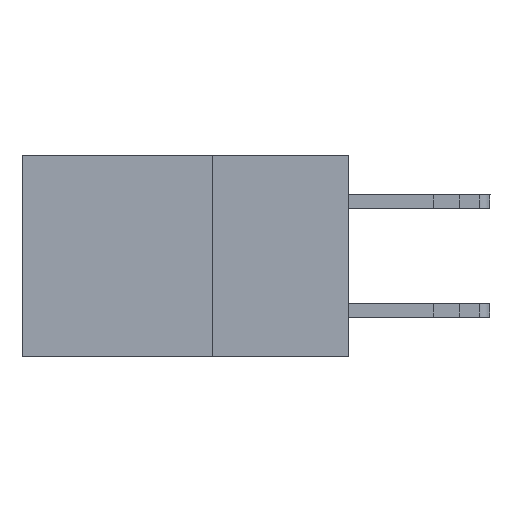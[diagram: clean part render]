
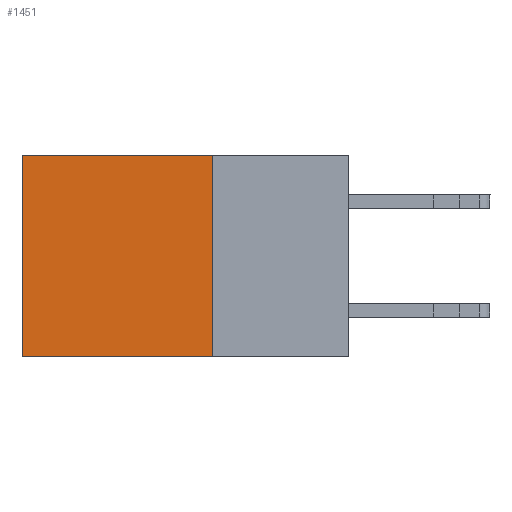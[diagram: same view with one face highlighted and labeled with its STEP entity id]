
A CAD part, left-side view. The second image highlights one B-rep face of the part: STEP entity #1451.
In plain terms, the highlighted planar face has unit normal (-1, 0, 0).
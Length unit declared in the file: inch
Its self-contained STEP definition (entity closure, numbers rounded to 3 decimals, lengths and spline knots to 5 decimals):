
#61 = VERTEX_POINT ( 'NONE', #7611 ) ;
#234 = VECTOR ( 'NONE', #950, 39.37008 ) ;
#636 = EDGE_LOOP ( 'NONE', ( #12539, #14292, #8505, #3517 ) ) ;
#950 = DIRECTION ( 'NONE',  ( 0., 0., -1. ) ) ;
#1048 = VECTOR ( 'NONE', #4160, 39.37008 ) ;
#1451 = ADVANCED_FACE ( 'NONE', ( #7456 ), #11274, .F. ) ;
#1726 = CARTESIAN_POINT ( 'NONE',  ( 0.298, 0.6, -0.37 ) ) ;
#2780 = VERTEX_POINT ( 'NONE', #1726 ) ;
#3517 = ORIENTED_EDGE ( 'NONE', *, *, #5756, .T. ) ;
#4160 = DIRECTION ( 'NONE',  ( 0., 1., 0. ) ) ;
#5051 = VECTOR ( 'NONE', #15753, 39.37008 ) ;
#5756 = EDGE_CURVE ( 'NONE', #9097, #61, #6914, .T. ) ;
#6095 = CARTESIAN_POINT ( 'NONE',  ( 0.298, 0.25, 0. ) ) ;
#6914 = LINE ( 'NONE', #16057, #1048 ) ;
#7456 = FACE_OUTER_BOUND ( 'NONE', #636, .T. ) ;
#7611 = CARTESIAN_POINT ( 'NONE',  ( 0.298, 0.6, 0. ) ) ;
#7722 = LINE ( 'NONE', #16698, #234 ) ;
#8208 = AXIS2_PLACEMENT_3D ( 'NONE', #6095, #13768, #8411 ) ;
#8411 = DIRECTION ( 'NONE',  ( 0., 0., -1. ) ) ;
#8505 = ORIENTED_EDGE ( 'NONE', *, *, #15843, .F. ) ;
#9097 = VERTEX_POINT ( 'NONE', #16712 ) ;
#9274 = VECTOR ( 'NONE', #11407, 39.37008 ) ;
#10507 = CARTESIAN_POINT ( 'NONE',  ( 0.298, 0.6, 0. ) ) ;
#10950 = CARTESIAN_POINT ( 'NONE',  ( 0.298, 0.25, -0.37 ) ) ;
#11274 = PLANE ( 'NONE',  #8208 ) ;
#11407 = DIRECTION ( 'NONE',  ( 0., 1., 0. ) ) ;
#12029 = VERTEX_POINT ( 'NONE', #10950 ) ;
#12471 = LINE ( 'NONE', #10507, #5051 ) ;
#12539 = ORIENTED_EDGE ( 'NONE', *, *, #12554, .T. ) ;
#12554 = EDGE_CURVE ( 'NONE', #61, #2780, #12471, .T. ) ;
#12704 = LINE ( 'NONE', #13902, #9274 ) ;
#13768 = DIRECTION ( 'NONE',  ( 1., 0., 0. ) ) ;
#13902 = CARTESIAN_POINT ( 'NONE',  ( 0.298, 0.25, -0.37 ) ) ;
#14292 = ORIENTED_EDGE ( 'NONE', *, *, #15449, .F. ) ;
#15449 = EDGE_CURVE ( 'NONE', #12029, #2780, #12704, .T. ) ;
#15753 = DIRECTION ( 'NONE',  ( 0., 0., -1. ) ) ;
#15843 = EDGE_CURVE ( 'NONE', #9097, #12029, #7722, .T. ) ;
#16057 = CARTESIAN_POINT ( 'NONE',  ( 0.298, 0.25, 0. ) ) ;
#16698 = CARTESIAN_POINT ( 'NONE',  ( 0.298, 0.25, 0. ) ) ;
#16712 = CARTESIAN_POINT ( 'NONE',  ( 0.298, 0.25, 0. ) ) ;
